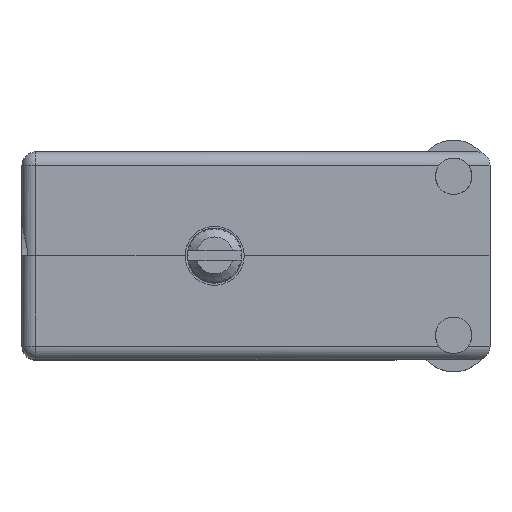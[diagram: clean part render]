
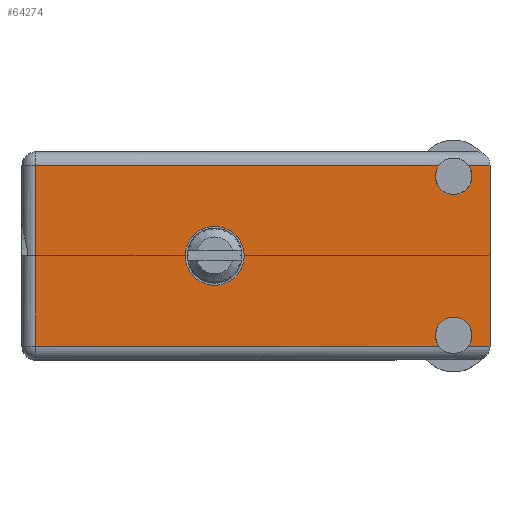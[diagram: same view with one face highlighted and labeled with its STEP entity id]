
A CAD part, top view. The second image highlights one B-rep face of the part: STEP entity #64274.
In plain terms, the highlighted face is planar.
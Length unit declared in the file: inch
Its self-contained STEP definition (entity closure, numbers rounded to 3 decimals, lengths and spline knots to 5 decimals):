
#760 = DIRECTION ( 'NONE',  ( 0., 1., 0. ) ) ;
#1541 = DIRECTION ( 'NONE',  ( 0., 1., 0. ) ) ;
#6613 = AXIS2_PLACEMENT_3D ( 'NONE', #122710, #21915, #67507 ) ;
#7256 = CARTESIAN_POINT ( 'NONE',  ( 0.8215, 0.806, 0.211 ) ) ;
#7571 = CARTESIAN_POINT ( 'NONE',  ( 0., 0.806, 0. ) ) ;
#9931 = LINE ( 'NONE', #90257, #101923 ) ;
#17103 = AXIS2_PLACEMENT_3D ( 'NONE', #7571, #155281, #183564 ) ;
#21915 = DIRECTION ( 'NONE',  ( 0., 1., 0. ) ) ;
#22607 = CARTESIAN_POINT ( 'NONE',  ( -0.6625, 0.806, -0.3105 ) ) ;
#24681 = ORIENTED_EDGE ( 'NONE', *, *, #51645, .F. ) ;
#29213 = LINE ( 'NONE', #22607, #88862 ) ;
#30526 = DIRECTION ( 'NONE',  ( 0., 0., 1. ) ) ;
#31677 = VERTEX_POINT ( 'NONE', #140616 ) ;
#32591 = ORIENTED_EDGE ( 'NONE', *, *, #180479, .T. ) ;
#32602 = ORIENTED_EDGE ( 'NONE', *, *, #78934, .F. ) ;
#32674 = CIRCLE ( 'NONE', #17103, 0.1015 ) ;
#35247 = ORIENTED_EDGE ( 'NONE', *, *, #154444, .T. ) ;
#38374 = EDGE_CURVE ( 'NONE', #125519, #31677, #32674, .T. ) ;
#40451 = DIRECTION ( 'NONE',  ( -1., 0., 0. ) ) ;
#41699 = DIRECTION ( 'NONE',  ( 0., 1., 0. ) ) ;
#42047 = DIRECTION ( 'NONE',  ( 1., 0., 0. ) ) ;
#43331 = VERTEX_POINT ( 'NONE', #153343 ) ;
#45071 = VECTOR ( 'NONE', #42047, 39.37008 ) ;
#48312 = AXIS2_PLACEMENT_3D ( 'NONE', #98156, #41699, #40451 ) ;
#50702 = VERTEX_POINT ( 'NONE', #67283 ) ;
#51645 = EDGE_CURVE ( 'NONE', #43331, #149785, #145205, .T. ) ;
#55522 = CARTESIAN_POINT ( 'NONE',  ( 0.9465, 0.806, 0.3105 ) ) ;
#56841 = EDGE_CURVE ( 'NONE', #77720, #114858, #189690, .T. ) ;
#59339 = DIRECTION ( 'NONE',  ( 0., 0., 1. ) ) ;
#60176 = LINE ( 'NONE', #147341, #113053 ) ;
#60985 = ORIENTED_EDGE ( 'NONE', *, *, #86957, .F. ) ;
#62374 = FACE_BOUND ( 'NONE', #143079, .T. ) ;
#63050 = DIRECTION ( 'NONE',  ( 0., 0., 1. ) ) ;
#64274 = ADVANCED_FACE ( 'NONE', ( #62374, #89872 ), #171374, .T. ) ;
#64995 = DIRECTION ( 'NONE',  ( -1., 0., 0. ) ) ;
#67283 = CARTESIAN_POINT ( 'NONE',  ( -0.6155, 0.806, -0.3105 ) ) ;
#67507 = DIRECTION ( 'NONE',  ( 0., 0., 1. ) ) ;
#67686 = CARTESIAN_POINT ( 'NONE',  ( 0.9465, 0.806, 0.3105 ) ) ;
#67907 = VECTOR ( 'NONE', #174340, 39.37008 ) ;
#69853 = AXIS2_PLACEMENT_3D ( 'NONE', #120159, #760, #161965 ) ;
#70686 = ORIENTED_EDGE ( 'NONE', *, *, #93818, .F. ) ;
#72908 = CARTESIAN_POINT ( 'NONE',  ( 0.8215, 0.806, -0.2735 ) ) ;
#77720 = VERTEX_POINT ( 'NONE', #81652 ) ;
#78934 = EDGE_CURVE ( 'NONE', #124162, #108096, #151135, .T. ) ;
#79006 = CIRCLE ( 'NONE', #84029, 0.1015 ) ;
#79458 = LINE ( 'NONE', #55522, #45071 ) ;
#80970 = EDGE_CURVE ( 'NONE', #120877, #114858, #79458, .T. ) ;
#81652 = CARTESIAN_POINT ( 'NONE',  ( 0.9465, 0.806, -0.3105 ) ) ;
#82786 = DIRECTION ( 'NONE',  ( -1., 0., 0. ) ) ;
#84029 = AXIS2_PLACEMENT_3D ( 'NONE', #172404, #84450, #187161 ) ;
#84450 = DIRECTION ( 'NONE',  ( 0., 1., 0. ) ) ;
#86270 = ORIENTED_EDGE ( 'NONE', *, *, #38374, .F. ) ;
#86957 = EDGE_CURVE ( 'NONE', #143462, #43331, #145959, .T. ) ;
#88862 = VECTOR ( 'NONE', #64995, 39.37008 ) ;
#89872 = FACE_OUTER_BOUND ( 'NONE', #120886, .T. ) ;
#90257 = CARTESIAN_POINT ( 'NONE',  ( 0.9465, 0.806, 0.3105 ) ) ;
#93818 = EDGE_CURVE ( 'NONE', #120877, #124162, #122092, .T. ) ;
#98156 = CARTESIAN_POINT ( 'NONE',  ( -0.6625, 0.806, -0.3575 ) ) ;
#101923 = VECTOR ( 'NONE', #117280, 39.37008 ) ;
#103131 = CARTESIAN_POINT ( 'NONE',  ( 0.77113, 0.806, 0.3105 ) ) ;
#107730 = VERTEX_POINT ( 'NONE', #148952 ) ;
#108096 = VERTEX_POINT ( 'NONE', #103131 ) ;
#113053 = VECTOR ( 'NONE', #59339, 39.37008 ) ;
#114858 = VERTEX_POINT ( 'NONE', #67686 ) ;
#117280 = DIRECTION ( 'NONE',  ( 1., 0., 0. ) ) ;
#120159 = CARTESIAN_POINT ( 'NONE',  ( 0.8215, 0.806, 0.2735 ) ) ;
#120668 = EDGE_CURVE ( 'NONE', #77720, #149785, #29213, .T. ) ;
#120877 = VERTEX_POINT ( 'NONE', #181864 ) ;
#120886 = EDGE_LOOP ( 'NONE', ( #153963, #32602, #70686, #173640, #168714, #154054, #24681, #60985, #35247, #32591 ) ) ;
#122092 = CIRCLE ( 'NONE', #6613, 0.0625 ) ;
#122710 = CARTESIAN_POINT ( 'NONE',  ( 0.8215, 0.806, 0.2735 ) ) ;
#123102 = LINE ( 'NONE', #156621, #141618 ) ;
#124162 = VERTEX_POINT ( 'NONE', #7256 ) ;
#125519 = VERTEX_POINT ( 'NONE', #154447 ) ;
#129394 = EDGE_CURVE ( 'NONE', #31677, #125519, #79006, .T. ) ;
#131084 = EDGE_CURVE ( 'NONE', #107730, #108096, #9931, .T. ) ;
#140616 = CARTESIAN_POINT ( 'NONE',  ( 0., 0.806, -0.1015 ) ) ;
#141618 = VECTOR ( 'NONE', #82786, 39.37008 ) ;
#141949 = CARTESIAN_POINT ( 'NONE',  ( 0.77113, 0.806, -0.3105 ) ) ;
#143079 = EDGE_LOOP ( 'NONE', ( #86270, #176366 ) ) ;
#143462 = VERTEX_POINT ( 'NONE', #141949 ) ;
#145205 = CIRCLE ( 'NONE', #167474, 0.0625 ) ;
#145959 = CIRCLE ( 'NONE', #164146, 0.0625 ) ;
#147341 = CARTESIAN_POINT ( 'NONE',  ( -0.6155, 0.806, -0.3575 ) ) ;
#148952 = CARTESIAN_POINT ( 'NONE',  ( -0.6155, 0.806, 0.3105 ) ) ;
#149785 = VERTEX_POINT ( 'NONE', #187993 ) ;
#151135 = CIRCLE ( 'NONE', #69853, 0.0625 ) ;
#153343 = CARTESIAN_POINT ( 'NONE',  ( 0.8215, 0.806, -0.211 ) ) ;
#153963 = ORIENTED_EDGE ( 'NONE', *, *, #131084, .T. ) ;
#154054 = ORIENTED_EDGE ( 'NONE', *, *, #120668, .T. ) ;
#154444 = EDGE_CURVE ( 'NONE', #143462, #50702, #123102, .T. ) ;
#154447 = CARTESIAN_POINT ( 'NONE',  ( 0., 0.806, 0.1015 ) ) ;
#155281 = DIRECTION ( 'NONE',  ( 0., 1., 0. ) ) ;
#156621 = CARTESIAN_POINT ( 'NONE',  ( -0.6625, 0.806, -0.3105 ) ) ;
#161965 = DIRECTION ( 'NONE',  ( 0., 0., 1. ) ) ;
#164146 = AXIS2_PLACEMENT_3D ( 'NONE', #72908, #1541, #30526 ) ;
#167474 = AXIS2_PLACEMENT_3D ( 'NONE', #176734, #179863, #63050 ) ;
#168714 = ORIENTED_EDGE ( 'NONE', *, *, #56841, .F. ) ;
#171374 = PLANE ( 'NONE',  #48312 ) ;
#172404 = CARTESIAN_POINT ( 'NONE',  ( 0., 0.806, 0. ) ) ;
#173640 = ORIENTED_EDGE ( 'NONE', *, *, #80970, .T. ) ;
#174340 = DIRECTION ( 'NONE',  ( 0., 0., 1. ) ) ;
#175588 = CARTESIAN_POINT ( 'NONE',  ( 0.9465, 0.806, 0.3575 ) ) ;
#176366 = ORIENTED_EDGE ( 'NONE', *, *, #129394, .F. ) ;
#176734 = CARTESIAN_POINT ( 'NONE',  ( 0.8215, 0.806, -0.2735 ) ) ;
#179863 = DIRECTION ( 'NONE',  ( 0., 1., 0. ) ) ;
#180479 = EDGE_CURVE ( 'NONE', #50702, #107730, #60176, .T. ) ;
#181864 = CARTESIAN_POINT ( 'NONE',  ( 0.87187, 0.806, 0.3105 ) ) ;
#183564 = DIRECTION ( 'NONE',  ( 0., 0., 1. ) ) ;
#187161 = DIRECTION ( 'NONE',  ( 0., 0., 1. ) ) ;
#187993 = CARTESIAN_POINT ( 'NONE',  ( 0.87187, 0.806, -0.3105 ) ) ;
#189690 = LINE ( 'NONE', #175588, #67907 ) ;
